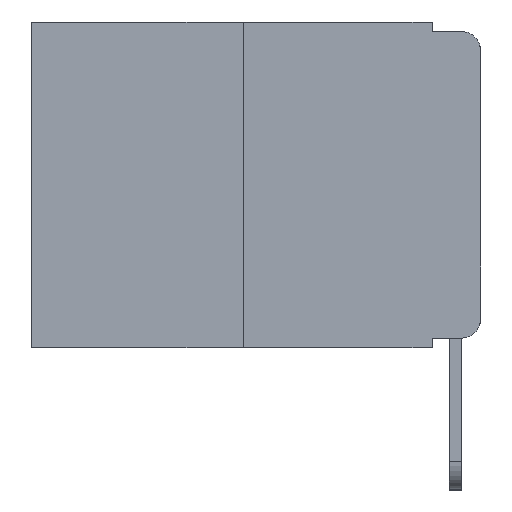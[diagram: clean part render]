
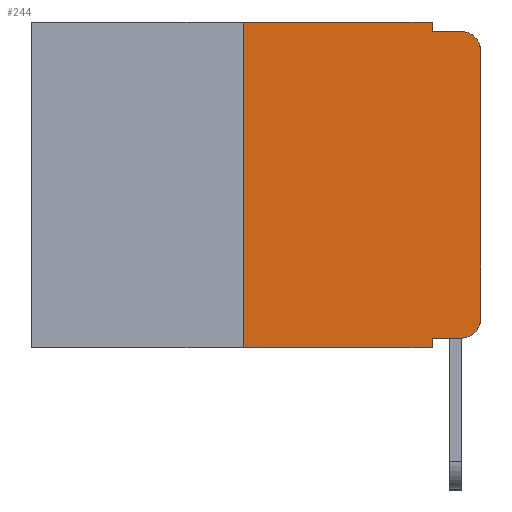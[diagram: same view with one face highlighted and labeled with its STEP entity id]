
A CAD part, left-side view. The second image highlights one B-rep face of the part: STEP entity #244.
In plain terms, the highlighted planar face has unit normal (-1, 0, 0).
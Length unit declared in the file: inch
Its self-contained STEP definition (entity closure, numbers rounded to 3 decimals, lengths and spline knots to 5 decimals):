
#28 = VERTEX_POINT ( 'NONE', #9670 ) ;
#200 = DIRECTION ( 'NONE',  ( 0., 0., -1. ) ) ;
#244 = ADVANCED_FACE ( 'NONE', ( #9409 ), #2417, .F. ) ;
#1086 = DIRECTION ( 'NONE',  ( 0., 0., -1. ) ) ;
#1097 = ORIENTED_EDGE ( 'NONE', *, *, #4149, .T. ) ;
#1100 = DIRECTION ( 'NONE',  ( 1., 0., 0. ) ) ;
#1259 = DIRECTION ( 'NONE',  ( 0., -1., 0. ) ) ;
#1330 = VERTEX_POINT ( 'NONE', #9118 ) ;
#1696 = CARTESIAN_POINT ( 'NONE',  ( 0., 0.051, 0. ) ) ;
#1793 = EDGE_CURVE ( 'NONE', #1330, #11815, #11450, .T. ) ;
#2219 = CARTESIAN_POINT ( 'NONE',  ( 0., 0.25, 0. ) ) ;
#2417 = PLANE ( 'NONE',  #12321 ) ;
#2498 = VERTEX_POINT ( 'NONE', #5542 ) ;
#2805 = ORIENTED_EDGE ( 'NONE', *, *, #14256, .F. ) ;
#3028 = DIRECTION ( 'NONE',  ( 0., 0., -1. ) ) ;
#3356 = CARTESIAN_POINT ( 'NONE',  ( 0., 0.02, -0.333 ) ) ;
#3425 = EDGE_LOOP ( 'NONE', ( #14909, #1097, #3430, #13451, #2805, #10720, #5500, #9235, #7513, #3522 ) ) ;
#3430 = ORIENTED_EDGE ( 'NONE', *, *, #7473, .F. ) ;
#3522 = ORIENTED_EDGE ( 'NONE', *, *, #13592, .T. ) ;
#3636 = CARTESIAN_POINT ( 'NONE',  ( 0., 0.473, 0. ) ) ;
#3725 = EDGE_CURVE ( 'NONE', #1330, #2498, #13666, .T. ) ;
#3789 = LINE ( 'NONE', #6261, #10047 ) ;
#4149 = EDGE_CURVE ( 'NONE', #13868, #10115, #7982, .T. ) ;
#4925 = CARTESIAN_POINT ( 'NONE',  ( 0., 0.02, -0.313 ) ) ;
#4964 = CARTESIAN_POINT ( 'NONE',  ( 0., 0.02, -0.03 ) ) ;
#4978 = DIRECTION ( 'NONE',  ( 0., 0., -1. ) ) ;
#4980 = DIRECTION ( 'NONE',  ( -1., 0., 0. ) ) ;
#5500 = ORIENTED_EDGE ( 'NONE', *, *, #1793, .T. ) ;
#5506 = CARTESIAN_POINT ( 'NONE',  ( 0., 0.473, -0.343 ) ) ;
#5542 = CARTESIAN_POINT ( 'NONE',  ( 0., 0.25, 0. ) ) ;
#5714 = VERTEX_POINT ( 'NONE', #15854 ) ;
#5720 = VECTOR ( 'NONE', #7129, 39.37008 ) ;
#5758 = CARTESIAN_POINT ( 'NONE',  ( 0., 0., -0.313 ) ) ;
#5883 = AXIS2_PLACEMENT_3D ( 'NONE', #4925, #13469, #6203 ) ;
#6162 = VECTOR ( 'NONE', #3028, 39.37008 ) ;
#6203 = DIRECTION ( 'NONE',  ( 0., 0., -1. ) ) ;
#6261 = CARTESIAN_POINT ( 'NONE',  ( 0., 0.051, 0. ) ) ;
#6844 = VERTEX_POINT ( 'NONE', #14943 ) ;
#7051 = CARTESIAN_POINT ( 'NONE',  ( 0., 0., 0. ) ) ;
#7129 = DIRECTION ( 'NONE',  ( 0., -1., 0. ) ) ;
#7258 = VECTOR ( 'NONE', #15967, 39.37008 ) ;
#7473 = EDGE_CURVE ( 'NONE', #28, #10115, #14989, .T. ) ;
#7513 = ORIENTED_EDGE ( 'NONE', *, *, #11989, .T. ) ;
#7680 = LINE ( 'NONE', #14151, #13721 ) ;
#7735 = EDGE_CURVE ( 'NONE', #8369, #13868, #14417, .T. ) ;
#7982 = CIRCLE ( 'NONE', #15658, 0.02 ) ;
#8012 = CARTESIAN_POINT ( 'NONE',  ( 0., 0.473, 0. ) ) ;
#8154 = VECTOR ( 'NONE', #14735, 39.37008 ) ;
#8369 = VERTEX_POINT ( 'NONE', #5758 ) ;
#9029 = CARTESIAN_POINT ( 'NONE',  ( 0., 0.051, -0.343 ) ) ;
#9118 = CARTESIAN_POINT ( 'NONE',  ( 0., 0.25, -0.343 ) ) ;
#9235 = ORIENTED_EDGE ( 'NONE', *, *, #10770, .F. ) ;
#9295 = EDGE_CURVE ( 'NONE', #6844, #28, #3789, .T. ) ;
#9409 = FACE_OUTER_BOUND ( 'NONE', #3425, .T. ) ;
#9670 = CARTESIAN_POINT ( 'NONE',  ( 0., 0.051, -0.01 ) ) ;
#9731 = VERTEX_POINT ( 'NONE', #3356 ) ;
#10047 = VECTOR ( 'NONE', #4978, 39.37008 ) ;
#10115 = VERTEX_POINT ( 'NONE', #10440 ) ;
#10440 = CARTESIAN_POINT ( 'NONE',  ( 0., 0.02, -0.01 ) ) ;
#10673 = VECTOR ( 'NONE', #13072, 39.37008 ) ;
#10720 = ORIENTED_EDGE ( 'NONE', *, *, #3725, .F. ) ;
#10770 = EDGE_CURVE ( 'NONE', #5714, #11815, #15816, .T. ) ;
#11380 = LINE ( 'NONE', #3636, #8154 ) ;
#11450 = LINE ( 'NONE', #5506, #5720 ) ;
#11596 = CIRCLE ( 'NONE', #5883, 0.02 ) ;
#11723 = DIRECTION ( 'NONE',  ( 0., -1., 0. ) ) ;
#11815 = VERTEX_POINT ( 'NONE', #9029 ) ;
#11989 = EDGE_CURVE ( 'NONE', #5714, #9731, #7680, .T. ) ;
#12174 = VECTOR ( 'NONE', #1259, 39.37008 ) ;
#12321 = AXIS2_PLACEMENT_3D ( 'NONE', #8012, #1100, #1086 ) ;
#13072 = DIRECTION ( 'NONE',  ( 0., 0., 1. ) ) ;
#13451 = ORIENTED_EDGE ( 'NONE', *, *, #9295, .F. ) ;
#13469 = DIRECTION ( 'NONE',  ( -1., 0., 0. ) ) ;
#13592 = EDGE_CURVE ( 'NONE', #9731, #8369, #11596, .T. ) ;
#13666 = LINE ( 'NONE', #2219, #7258 ) ;
#13721 = VECTOR ( 'NONE', #11723, 39.37008 ) ;
#13868 = VERTEX_POINT ( 'NONE', #15209 ) ;
#14151 = CARTESIAN_POINT ( 'NONE',  ( 0., 0.051, -0.333 ) ) ;
#14256 = EDGE_CURVE ( 'NONE', #2498, #6844, #11380, .T. ) ;
#14417 = LINE ( 'NONE', #7051, #10673 ) ;
#14735 = DIRECTION ( 'NONE',  ( 0., -1., 0. ) ) ;
#14909 = ORIENTED_EDGE ( 'NONE', *, *, #7735, .T. ) ;
#14943 = CARTESIAN_POINT ( 'NONE',  ( 0., 0.051, 0. ) ) ;
#14975 = CARTESIAN_POINT ( 'NONE',  ( 0., 0.051, -0.01 ) ) ;
#14989 = LINE ( 'NONE', #14975, #12174 ) ;
#15209 = CARTESIAN_POINT ( 'NONE',  ( 0., 0., -0.03 ) ) ;
#15658 = AXIS2_PLACEMENT_3D ( 'NONE', #4964, #4980, #200 ) ;
#15816 = LINE ( 'NONE', #1696, #6162 ) ;
#15854 = CARTESIAN_POINT ( 'NONE',  ( 0., 0.051, -0.333 ) ) ;
#15967 = DIRECTION ( 'NONE',  ( 0., 0., 1. ) ) ;
